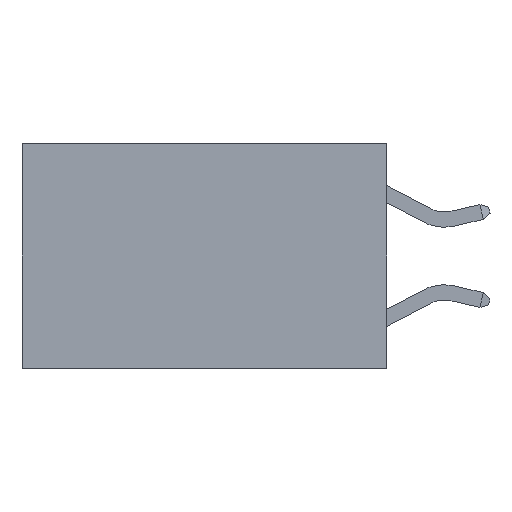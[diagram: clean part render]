
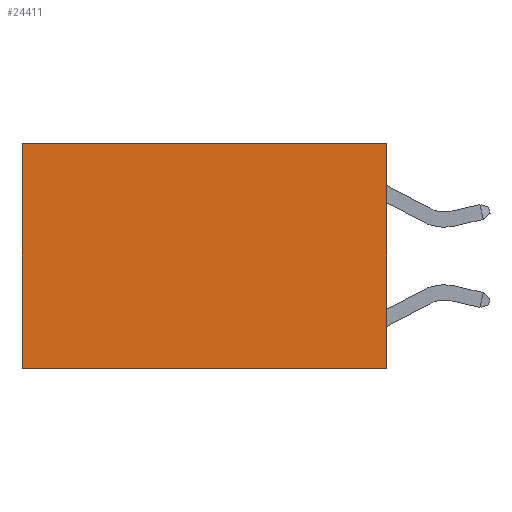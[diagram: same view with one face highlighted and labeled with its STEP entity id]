
A CAD part, left-side view. The second image highlights one B-rep face of the part: STEP entity #24411.
In plain terms, the highlighted planar face has unit normal (-1, 0, 0).
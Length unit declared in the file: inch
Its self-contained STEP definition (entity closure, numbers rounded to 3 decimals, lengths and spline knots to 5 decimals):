
#1654 = ORIENTED_EDGE ( 'NONE', *, *, #2514, .T. ) ;
#1857 = EDGE_CURVE ( 'NONE', #9821, #24152, #3771, .T. ) ;
#2514 = EDGE_CURVE ( 'NONE', #9821, #8138, #23947, .T. ) ;
#3057 = VECTOR ( 'NONE', #29716, 39.37008 ) ;
#3771 = LINE ( 'NONE', #13195, #3057 ) ;
#4475 = CARTESIAN_POINT ( 'NONE',  ( 0.2625, 0.6, 0. ) ) ;
#5883 = EDGE_CURVE ( 'NONE', #24152, #18407, #13732, .T. ) ;
#6498 = CARTESIAN_POINT ( 'NONE',  ( 0.2625, 0., -0.37 ) ) ;
#8015 = PLANE ( 'NONE',  #22849 ) ;
#8138 = VERTEX_POINT ( 'NONE', #24955 ) ;
#9088 = DIRECTION ( 'NONE',  ( 0., 1., 0. ) ) ;
#9821 = VERTEX_POINT ( 'NONE', #20066 ) ;
#9887 = DIRECTION ( 'NONE',  ( 0., 1., 0. ) ) ;
#11415 = CARTESIAN_POINT ( 'NONE',  ( 0.2625, 0., -0.37 ) ) ;
#12200 = CARTESIAN_POINT ( 'NONE',  ( 0.2625, 0., 0. ) ) ;
#13195 = CARTESIAN_POINT ( 'NONE',  ( 0.2625, 0., 0. ) ) ;
#13732 = LINE ( 'NONE', #11415, #29541 ) ;
#16781 = EDGE_LOOP ( 'NONE', ( #18617, #26848, #20656, #1654 ) ) ;
#17457 = CARTESIAN_POINT ( 'NONE',  ( 0.2625, 0., 0. ) ) ;
#17766 = DIRECTION ( 'NONE',  ( 1., 0., 0. ) ) ;
#18407 = VERTEX_POINT ( 'NONE', #28661 ) ;
#18617 = ORIENTED_EDGE ( 'NONE', *, *, #27958, .T. ) ;
#19772 = FACE_OUTER_BOUND ( 'NONE', #16781, .T. ) ;
#20066 = CARTESIAN_POINT ( 'NONE',  ( 0.2625, 0., 0. ) ) ;
#20406 = LINE ( 'NONE', #4475, #25836 ) ;
#20534 = DIRECTION ( 'NONE',  ( 0., 0., -1. ) ) ;
#20656 = ORIENTED_EDGE ( 'NONE', *, *, #1857, .F. ) ;
#20855 = DIRECTION ( 'NONE',  ( 0., 0., -1. ) ) ;
#22849 = AXIS2_PLACEMENT_3D ( 'NONE', #17457, #17766, #20534 ) ;
#22973 = VECTOR ( 'NONE', #9887, 39.37008 ) ;
#23947 = LINE ( 'NONE', #12200, #22973 ) ;
#24152 = VERTEX_POINT ( 'NONE', #6498 ) ;
#24411 = ADVANCED_FACE ( 'NONE', ( #19772 ), #8015, .F. ) ;
#24955 = CARTESIAN_POINT ( 'NONE',  ( 0.2625, 0.6, 0. ) ) ;
#25836 = VECTOR ( 'NONE', #20855, 39.37008 ) ;
#26848 = ORIENTED_EDGE ( 'NONE', *, *, #5883, .F. ) ;
#27958 = EDGE_CURVE ( 'NONE', #8138, #18407, #20406, .T. ) ;
#28661 = CARTESIAN_POINT ( 'NONE',  ( 0.2625, 0.6, -0.37 ) ) ;
#29541 = VECTOR ( 'NONE', #9088, 39.37008 ) ;
#29716 = DIRECTION ( 'NONE',  ( 0., 0., -1. ) ) ;
